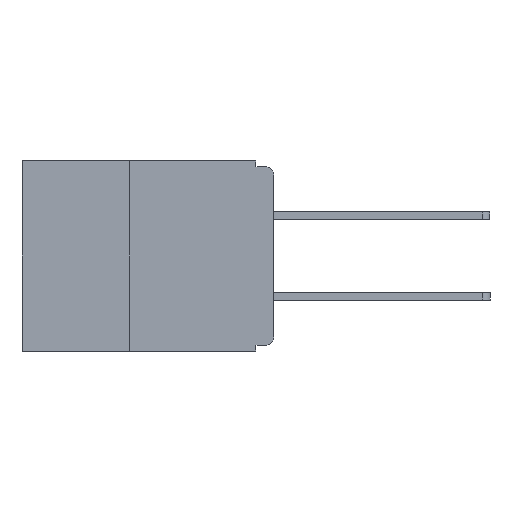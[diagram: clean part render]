
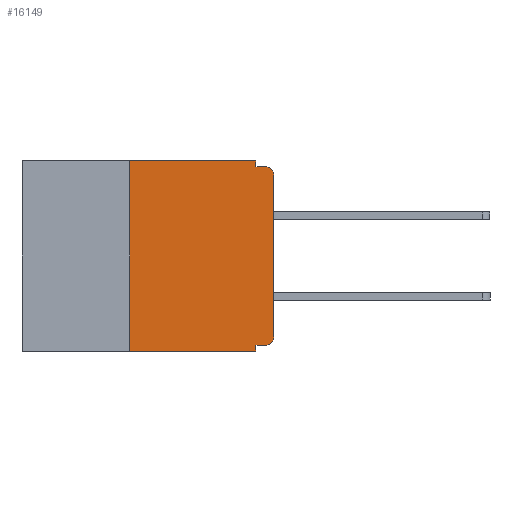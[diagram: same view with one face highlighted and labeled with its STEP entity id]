
A CAD part, left-side view. The second image highlights one B-rep face of the part: STEP entity #16149.
In plain terms, the highlighted planar face has unit normal (-1, 0, 0).
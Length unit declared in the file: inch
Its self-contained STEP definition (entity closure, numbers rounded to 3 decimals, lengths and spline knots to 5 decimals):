
#1093 = VECTOR ( 'NONE', #6856, 39.37008 ) ;
#1173 = CARTESIAN_POINT ( 'NONE',  ( 0., 0.031, 0. ) ) ;
#1528 = CARTESIAN_POINT ( 'NONE',  ( 0., 0., 0. ) ) ;
#1612 = EDGE_CURVE ( 'NONE', #17794, #23753, #23961, .T. ) ;
#1679 = ORIENTED_EDGE ( 'NONE', *, *, #22881, .F. ) ;
#2305 = EDGE_LOOP ( 'NONE', ( #6184, #21170, #7487, #30155, #6213, #1679, #32134, #2960, #11701, #33327 ) ) ;
#2743 = DIRECTION ( 'NONE',  ( 0., 1., 0. ) ) ;
#2960 = ORIENTED_EDGE ( 'NONE', *, *, #1612, .F. ) ;
#5172 = DIRECTION ( 'NONE',  ( 0., 0., 1. ) ) ;
#5265 = VERTEX_POINT ( 'NONE', #19514 ) ;
#6184 = ORIENTED_EDGE ( 'NONE', *, *, #28463, .T. ) ;
#6213 = ORIENTED_EDGE ( 'NONE', *, *, #18245, .F. ) ;
#6834 = EDGE_CURVE ( 'NONE', #19133, #32019, #7064, .T. ) ;
#6856 = DIRECTION ( 'NONE',  ( 0., 0., 1. ) ) ;
#7064 = CIRCLE ( 'NONE', #15456, 0.015 ) ;
#7417 = CARTESIAN_POINT ( 'NONE',  ( 0., 0.031, -0.33 ) ) ;
#7487 = ORIENTED_EDGE ( 'NONE', *, *, #9705, .F. ) ;
#8470 = PLANE ( 'NONE',  #25558 ) ;
#9072 = VECTOR ( 'NONE', #16136, 39.37008 ) ;
#9684 = CARTESIAN_POINT ( 'NONE',  ( 0., 0.25, -0.33 ) ) ;
#9705 = EDGE_CURVE ( 'NONE', #15559, #32019, #27381, .T. ) ;
#10051 = DIRECTION ( 'NONE',  ( 0., -1., 0. ) ) ;
#10270 = VECTOR ( 'NONE', #11832, 39.37008 ) ;
#10854 = CARTESIAN_POINT ( 'NONE',  ( 0., 0.015, -0.01 ) ) ;
#10907 = EDGE_CURVE ( 'NONE', #26083, #17794, #19166, .T. ) ;
#11172 = DIRECTION ( 'NONE',  ( 1., 0., 0. ) ) ;
#11550 = CARTESIAN_POINT ( 'NONE',  ( 0., 0.031, -0.01 ) ) ;
#11701 = ORIENTED_EDGE ( 'NONE', *, *, #10907, .F. ) ;
#11832 = DIRECTION ( 'NONE',  ( 0., -1., 0. ) ) ;
#12545 = CARTESIAN_POINT ( 'NONE',  ( 0., 0.031, -0.32 ) ) ;
#12557 = VECTOR ( 'NONE', #10051, 39.37008 ) ;
#12633 = CARTESIAN_POINT ( 'NONE',  ( 0., 0.015, -0.305 ) ) ;
#13222 = CARTESIAN_POINT ( 'NONE',  ( 0., 0.25, -0.33 ) ) ;
#13967 = LINE ( 'NONE', #1173, #28152 ) ;
#14651 = CARTESIAN_POINT ( 'NONE',  ( 0., 0., -0.305 ) ) ;
#15347 = DIRECTION ( 'NONE',  ( 0., 0., -1. ) ) ;
#15453 = VECTOR ( 'NONE', #16298, 39.37008 ) ;
#15456 = AXIS2_PLACEMENT_3D ( 'NONE', #27126, #27087, #27045 ) ;
#15559 = VERTEX_POINT ( 'NONE', #11550 ) ;
#15642 = EDGE_CURVE ( 'NONE', #5265, #15559, #13967, .T. ) ;
#16136 = DIRECTION ( 'NONE',  ( 0., 0., -1. ) ) ;
#16149 = ADVANCED_FACE ( 'NONE', ( #19559 ), #8470, .F. ) ;
#16298 = DIRECTION ( 'NONE',  ( 0., -1., 0. ) ) ;
#17400 = CARTESIAN_POINT ( 'NONE',  ( 0., 0.031, -0.33 ) ) ;
#17794 = VERTEX_POINT ( 'NONE', #12545 ) ;
#18245 = EDGE_CURVE ( 'NONE', #31394, #5265, #31176, .T. ) ;
#19133 = VERTEX_POINT ( 'NONE', #26143 ) ;
#19166 = LINE ( 'NONE', #28950, #31317 ) ;
#19514 = CARTESIAN_POINT ( 'NONE',  ( 0., 0.031, 0. ) ) ;
#19559 = FACE_OUTER_BOUND ( 'NONE', #2305, .T. ) ;
#20585 = EDGE_CURVE ( 'NONE', #30217, #23753, #22432, .T. ) ;
#21170 = ORIENTED_EDGE ( 'NONE', *, *, #6834, .T. ) ;
#22395 = DIRECTION ( 'NONE',  ( 0., 0., -1. ) ) ;
#22432 = LINE ( 'NONE', #26693, #15453 ) ;
#22718 = EDGE_CURVE ( 'NONE', #26083, #27620, #23919, .T. ) ;
#22881 = EDGE_CURVE ( 'NONE', #30217, #31394, #31975, .T. ) ;
#23753 = VERTEX_POINT ( 'NONE', #17400 ) ;
#23919 = CIRCLE ( 'NONE', #28379, 0.015 ) ;
#23961 = LINE ( 'NONE', #7417, #9072 ) ;
#24192 = CARTESIAN_POINT ( 'NONE',  ( 0., 0.437, 0. ) ) ;
#25118 = VECTOR ( 'NONE', #5172, 39.37008 ) ;
#25558 = AXIS2_PLACEMENT_3D ( 'NONE', #24192, #11172, #29569 ) ;
#26083 = VERTEX_POINT ( 'NONE', #26308 ) ;
#26143 = CARTESIAN_POINT ( 'NONE',  ( 0., 0., -0.025 ) ) ;
#26308 = CARTESIAN_POINT ( 'NONE',  ( 0., 0.015, -0.32 ) ) ;
#26693 = CARTESIAN_POINT ( 'NONE',  ( 0., 0.437, -0.33 ) ) ;
#27045 = DIRECTION ( 'NONE',  ( 0., 0., -1. ) ) ;
#27087 = DIRECTION ( 'NONE',  ( -1., 0., 0. ) ) ;
#27126 = CARTESIAN_POINT ( 'NONE',  ( 0., 0.015, -0.025 ) ) ;
#27381 = LINE ( 'NONE', #28459, #12557 ) ;
#27620 = VERTEX_POINT ( 'NONE', #14651 ) ;
#28152 = VECTOR ( 'NONE', #22395, 39.37008 ) ;
#28379 = AXIS2_PLACEMENT_3D ( 'NONE', #12633, #30962, #15347 ) ;
#28459 = CARTESIAN_POINT ( 'NONE',  ( 0., 0., -0.01 ) ) ;
#28463 = EDGE_CURVE ( 'NONE', #27620, #19133, #29223, .T. ) ;
#28950 = CARTESIAN_POINT ( 'NONE',  ( 0., 0., -0.32 ) ) ;
#29061 = CARTESIAN_POINT ( 'NONE',  ( 0., 0.25, 0. ) ) ;
#29223 = LINE ( 'NONE', #1528, #1093 ) ;
#29569 = DIRECTION ( 'NONE',  ( 0., 0., -1. ) ) ;
#30155 = ORIENTED_EDGE ( 'NONE', *, *, #15642, .F. ) ;
#30217 = VERTEX_POINT ( 'NONE', #9684 ) ;
#30962 = DIRECTION ( 'NONE',  ( -1., 0., 0. ) ) ;
#31176 = LINE ( 'NONE', #32719, #10270 ) ;
#31317 = VECTOR ( 'NONE', #2743, 39.37008 ) ;
#31394 = VERTEX_POINT ( 'NONE', #29061 ) ;
#31975 = LINE ( 'NONE', #13222, #25118 ) ;
#32019 = VERTEX_POINT ( 'NONE', #10854 ) ;
#32134 = ORIENTED_EDGE ( 'NONE', *, *, #20585, .T. ) ;
#32719 = CARTESIAN_POINT ( 'NONE',  ( 0., 0.437, 0. ) ) ;
#33327 = ORIENTED_EDGE ( 'NONE', *, *, #22718, .T. ) ;
